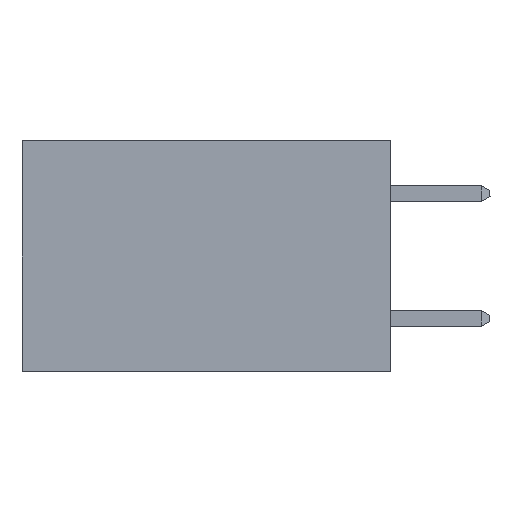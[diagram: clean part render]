
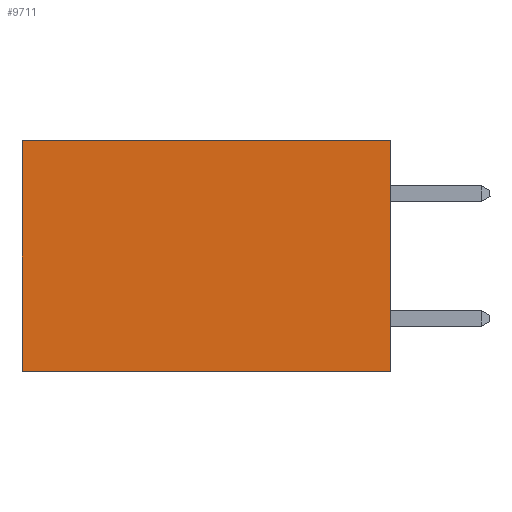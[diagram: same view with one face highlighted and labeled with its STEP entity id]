
A CAD part, left-side view. The second image highlights one B-rep face of the part: STEP entity #9711.
In plain terms, the highlighted planar face has unit normal (-1, 0, 0).
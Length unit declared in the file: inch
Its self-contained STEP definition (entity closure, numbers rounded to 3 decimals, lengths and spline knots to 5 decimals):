
#1138 = LINE ( 'NONE', #3716, #5085 ) ;
#1352 = CARTESIAN_POINT ( 'NONE',  ( 0.277, 0., -0.37 ) ) ;
#1693 = ORIENTED_EDGE ( 'NONE', *, *, #13505, .F. ) ;
#2267 = VECTOR ( 'NONE', #12729, 39.37008 ) ;
#2528 = AXIS2_PLACEMENT_3D ( 'NONE', #1352, #23582, #5982 ) ;
#2908 = CARTESIAN_POINT ( 'NONE',  ( 0.277, 0., 0. ) ) ;
#3716 = CARTESIAN_POINT ( 'NONE',  ( 0.277, 0., 0. ) ) ;
#3720 = EDGE_CURVE ( 'NONE', #22335, #16498, #4130, .T. ) ;
#4130 = LINE ( 'NONE', #10918, #10374 ) ;
#4926 = FACE_OUTER_BOUND ( 'NONE', #10974, .T. ) ;
#5085 = VECTOR ( 'NONE', #5670, 39.37008 ) ;
#5481 = ORIENTED_EDGE ( 'NONE', *, *, #12709, .F. ) ;
#5617 = VERTEX_POINT ( 'NONE', #13897 ) ;
#5670 = DIRECTION ( 'NONE',  ( 0., 1., 0. ) ) ;
#5982 = DIRECTION ( 'NONE',  ( 0., 0., -1. ) ) ;
#6266 = VECTOR ( 'NONE', #8590, 39.37008 ) ;
#6702 = CARTESIAN_POINT ( 'NONE',  ( 0.277, 0., -0.37 ) ) ;
#6731 = VERTEX_POINT ( 'NONE', #2908 ) ;
#7236 = ORIENTED_EDGE ( 'NONE', *, *, #3720, .T. ) ;
#8590 = DIRECTION ( 'NONE',  ( 0., 1., 0. ) ) ;
#9711 = ADVANCED_FACE ( 'NONE', ( #4926 ), #23609, .F. ) ;
#10374 = VECTOR ( 'NONE', #24046, 39.37008 ) ;
#10918 = CARTESIAN_POINT ( 'NONE',  ( 0.277, 0.59, -0.37 ) ) ;
#10974 = EDGE_LOOP ( 'NONE', ( #7236, #5481, #1693, #16633 ) ) ;
#11173 = CARTESIAN_POINT ( 'NONE',  ( 0.277, 0.59, 0. ) ) ;
#12709 = EDGE_CURVE ( 'NONE', #5617, #16498, #21054, .T. ) ;
#12729 = DIRECTION ( 'NONE',  ( 0., 0., -1. ) ) ;
#13505 = EDGE_CURVE ( 'NONE', #6731, #5617, #17275, .T. ) ;
#13897 = CARTESIAN_POINT ( 'NONE',  ( 0.277, 0., -0.37 ) ) ;
#16498 = VERTEX_POINT ( 'NONE', #21428 ) ;
#16633 = ORIENTED_EDGE ( 'NONE', *, *, #22363, .T. ) ;
#17275 = LINE ( 'NONE', #18121, #2267 ) ;
#18121 = CARTESIAN_POINT ( 'NONE',  ( 0.277, 0., -0.37 ) ) ;
#21054 = LINE ( 'NONE', #6702, #6266 ) ;
#21428 = CARTESIAN_POINT ( 'NONE',  ( 0.277, 0.59, -0.37 ) ) ;
#22335 = VERTEX_POINT ( 'NONE', #11173 ) ;
#22363 = EDGE_CURVE ( 'NONE', #6731, #22335, #1138, .T. ) ;
#23582 = DIRECTION ( 'NONE',  ( 1., 0., 0. ) ) ;
#23609 = PLANE ( 'NONE',  #2528 ) ;
#24046 = DIRECTION ( 'NONE',  ( 0., 0., -1. ) ) ;
